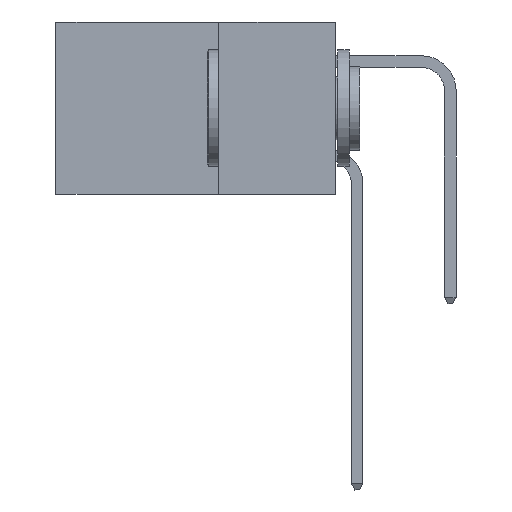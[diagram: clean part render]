
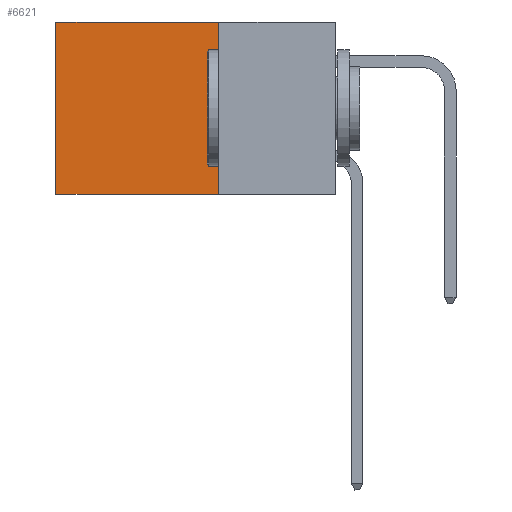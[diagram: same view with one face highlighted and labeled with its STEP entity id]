
A CAD part, left-side view. The second image highlights one B-rep face of the part: STEP entity #6621.
In plain terms, the highlighted planar face has unit normal (-1, 0, 0).
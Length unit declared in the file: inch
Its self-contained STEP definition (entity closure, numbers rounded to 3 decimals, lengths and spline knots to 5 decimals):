
#890 = VERTEX_POINT ( 'NONE', #10402 ) ;
#1296 = VECTOR ( 'NONE', #11872, 39.37008 ) ;
#1298 = ORIENTED_EDGE ( 'NONE', *, *, #7901, .T. ) ;
#2661 = VECTOR ( 'NONE', #11095, 39.37008 ) ;
#2824 = PLANE ( 'NONE',  #12308 ) ;
#3136 = EDGE_LOOP ( 'NONE', ( #1298, #10147, #9387, #7962 ) ) ;
#3713 = CARTESIAN_POINT ( 'NONE',  ( 0.2875, 0.25, 0. ) ) ;
#4854 = CARTESIAN_POINT ( 'NONE',  ( 0.2875, 0.25, -0.37 ) ) ;
#4999 = CARTESIAN_POINT ( 'NONE',  ( 0.2875, 0.25, 0. ) ) ;
#5044 = CARTESIAN_POINT ( 'NONE',  ( 0.2875, 0.25, 0. ) ) ;
#5261 = CARTESIAN_POINT ( 'NONE',  ( 0.2875, 0.6, -0.37 ) ) ;
#6102 = LINE ( 'NONE', #4854, #1296 ) ;
#6621 = ADVANCED_FACE ( 'NONE', ( #9064 ), #2824, .F. ) ;
#6720 = EDGE_CURVE ( 'NONE', #11492, #890, #10750, .T. ) ;
#6941 = DIRECTION ( 'NONE',  ( 0., 0., -1. ) ) ;
#7901 = EDGE_CURVE ( 'NONE', #13047, #8618, #10579, .T. ) ;
#7962 = ORIENTED_EDGE ( 'NONE', *, *, #11708, .T. ) ;
#8254 = VECTOR ( 'NONE', #11153, 39.37008 ) ;
#8533 = CARTESIAN_POINT ( 'NONE',  ( 0.2875, 0.6, 0. ) ) ;
#8618 = VERTEX_POINT ( 'NONE', #5261 ) ;
#8885 = VECTOR ( 'NONE', #9172, 39.37008 ) ;
#8960 = CARTESIAN_POINT ( 'NONE',  ( 0.2875, 0.25, 0. ) ) ;
#9064 = FACE_OUTER_BOUND ( 'NONE', #3136, .T. ) ;
#9172 = DIRECTION ( 'NONE',  ( 0., 1., 0. ) ) ;
#9387 = ORIENTED_EDGE ( 'NONE', *, *, #6720, .F. ) ;
#10147 = ORIENTED_EDGE ( 'NONE', *, *, #12142, .F. ) ;
#10183 = CARTESIAN_POINT ( 'NONE',  ( 0.2875, 0.6, 0. ) ) ;
#10402 = CARTESIAN_POINT ( 'NONE',  ( 0.2875, 0.25, -0.37 ) ) ;
#10579 = LINE ( 'NONE', #10183, #8254 ) ;
#10750 = LINE ( 'NONE', #4999, #2661 ) ;
#11095 = DIRECTION ( 'NONE',  ( 0., 0., -1. ) ) ;
#11153 = DIRECTION ( 'NONE',  ( 0., 0., -1. ) ) ;
#11481 = LINE ( 'NONE', #5044, #8885 ) ;
#11492 = VERTEX_POINT ( 'NONE', #3713 ) ;
#11708 = EDGE_CURVE ( 'NONE', #11492, #13047, #11481, .T. ) ;
#11872 = DIRECTION ( 'NONE',  ( 0., 1., 0. ) ) ;
#12142 = EDGE_CURVE ( 'NONE', #890, #8618, #6102, .T. ) ;
#12308 = AXIS2_PLACEMENT_3D ( 'NONE', #8960, #12855, #6941 ) ;
#12855 = DIRECTION ( 'NONE',  ( 1., 0., 0. ) ) ;
#13047 = VERTEX_POINT ( 'NONE', #8533 ) ;
